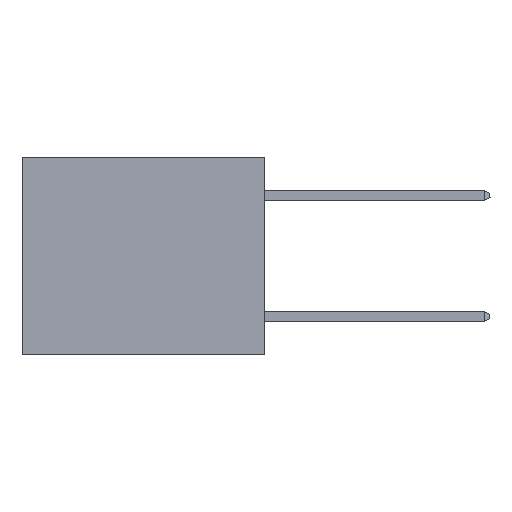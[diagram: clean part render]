
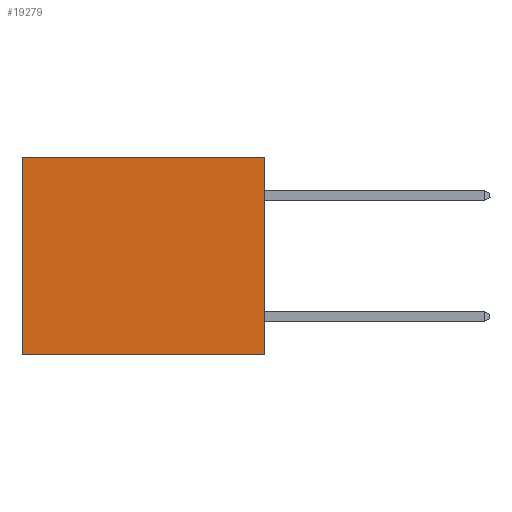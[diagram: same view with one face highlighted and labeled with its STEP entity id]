
A CAD part, left-side view. The second image highlights one B-rep face of the part: STEP entity #19279.
In plain terms, the highlighted planar face has unit normal (-1, 0, 0).
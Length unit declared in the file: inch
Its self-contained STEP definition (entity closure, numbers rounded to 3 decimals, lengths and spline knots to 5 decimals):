
#1008 = ORIENTED_EDGE ( 'NONE', *, *, #16525, .F. ) ;
#2937 = LINE ( 'NONE', #18235, #13335 ) ;
#4060 = ORIENTED_EDGE ( 'NONE', *, *, #20373, .T. ) ;
#4349 = DIRECTION ( 'NONE',  ( 0., 1., 0. ) ) ;
#4444 = EDGE_LOOP ( 'NONE', ( #16472, #1008, #11190, #4060 ) ) ;
#5053 = VECTOR ( 'NONE', #13870, 39.37008 ) ;
#6642 = DIRECTION ( 'NONE',  ( 0., 0., -1. ) ) ;
#7303 = EDGE_CURVE ( 'NONE', #10432, #20178, #2937, .T. ) ;
#7646 = VERTEX_POINT ( 'NONE', #12433 ) ;
#9263 = CARTESIAN_POINT ( 'NONE',  ( 0.3165, 0., -0.49 ) ) ;
#10432 = VERTEX_POINT ( 'NONE', #11655 ) ;
#10677 = VECTOR ( 'NONE', #13934, 39.37008 ) ;
#10716 = FACE_OUTER_BOUND ( 'NONE', #4444, .T. ) ;
#11190 = ORIENTED_EDGE ( 'NONE', *, *, #18628, .F. ) ;
#11655 = CARTESIAN_POINT ( 'NONE',  ( 0.3165, 0.6, 0. ) ) ;
#12433 = CARTESIAN_POINT ( 'NONE',  ( 0.3165, 0., 0. ) ) ;
#12662 = VECTOR ( 'NONE', #4349, 39.37008 ) ;
#12929 = LINE ( 'NONE', #9263, #12662 ) ;
#13028 = LINE ( 'NONE', #16908, #10677 ) ;
#13099 = LINE ( 'NONE', #20569, #5053 ) ;
#13335 = VECTOR ( 'NONE', #6642, 39.37008 ) ;
#13870 = DIRECTION ( 'NONE',  ( 0., 0., -1. ) ) ;
#13934 = DIRECTION ( 'NONE',  ( 0., 1., 0. ) ) ;
#15207 = CARTESIAN_POINT ( 'NONE',  ( 0.3165, 0., -0.49 ) ) ;
#15298 = DIRECTION ( 'NONE',  ( 0., 0., -1. ) ) ;
#15457 = CARTESIAN_POINT ( 'NONE',  ( 0.3165, 0., -0.49 ) ) ;
#16472 = ORIENTED_EDGE ( 'NONE', *, *, #7303, .T. ) ;
#16525 = EDGE_CURVE ( 'NONE', #18919, #20178, #12929, .T. ) ;
#16908 = CARTESIAN_POINT ( 'NONE',  ( 0.3165, 0., 0. ) ) ;
#18235 = CARTESIAN_POINT ( 'NONE',  ( 0.3165, 0.6, -0.49 ) ) ;
#18628 = EDGE_CURVE ( 'NONE', #7646, #18919, #13099, .T. ) ;
#18884 = DIRECTION ( 'NONE',  ( 1., 0., 0. ) ) ;
#18919 = VERTEX_POINT ( 'NONE', #15207 ) ;
#19279 = ADVANCED_FACE ( 'NONE', ( #10716 ), #20352, .F. ) ;
#20178 = VERTEX_POINT ( 'NONE', #20206 ) ;
#20206 = CARTESIAN_POINT ( 'NONE',  ( 0.3165, 0.6, -0.49 ) ) ;
#20352 = PLANE ( 'NONE',  #20381 ) ;
#20373 = EDGE_CURVE ( 'NONE', #7646, #10432, #13028, .T. ) ;
#20381 = AXIS2_PLACEMENT_3D ( 'NONE', #15457, #18884, #15298 ) ;
#20569 = CARTESIAN_POINT ( 'NONE',  ( 0.3165, 0., -0.49 ) ) ;
